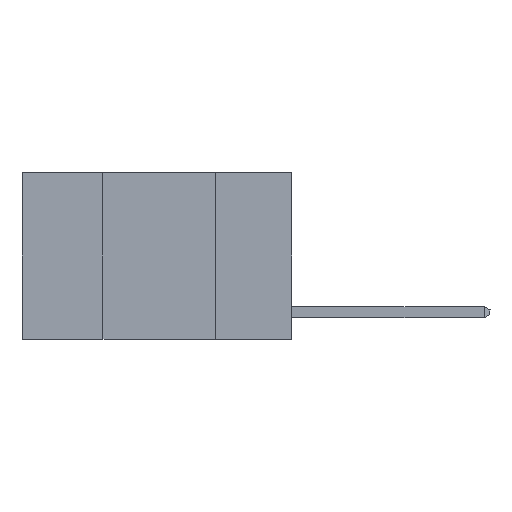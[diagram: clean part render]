
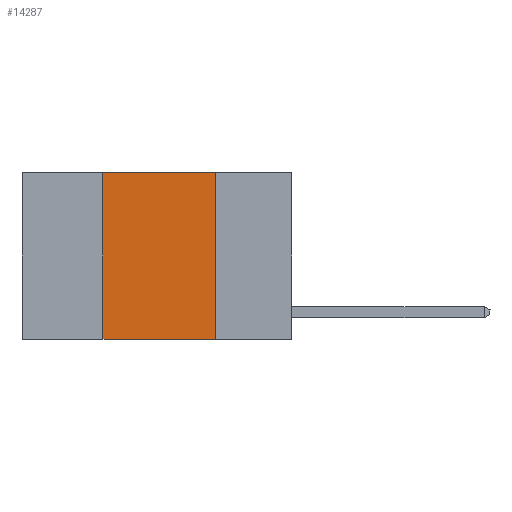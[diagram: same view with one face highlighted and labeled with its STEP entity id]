
A CAD part, left-side view. The second image highlights one B-rep face of the part: STEP entity #14287.
In plain terms, the highlighted planar face has unit normal (-1, 0, 0).
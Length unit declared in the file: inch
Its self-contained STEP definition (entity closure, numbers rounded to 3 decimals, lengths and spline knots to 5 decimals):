
#837 = EDGE_LOOP ( 'NONE', ( #17933, #16946, #6450, #17273 ) ) ;
#1262 = VECTOR ( 'NONE', #12781, 39.37008 ) ;
#1376 = VERTEX_POINT ( 'NONE', #6701 ) ;
#1674 = CARTESIAN_POINT ( 'NONE',  ( 0., 0.42, 0. ) ) ;
#2079 = DIRECTION ( 'NONE',  ( 0., -1., 0. ) ) ;
#2523 = DIRECTION ( 'NONE',  ( 0., -1., 0. ) ) ;
#2656 = VECTOR ( 'NONE', #2523, 39.37008 ) ;
#2995 = VERTEX_POINT ( 'NONE', #4851 ) ;
#3173 = CARTESIAN_POINT ( 'NONE',  ( 0., 0.6, 0. ) ) ;
#4442 = FACE_OUTER_BOUND ( 'NONE', #837, .T. ) ;
#4524 = CARTESIAN_POINT ( 'NONE',  ( 0., 0.17, 0. ) ) ;
#4851 = CARTESIAN_POINT ( 'NONE',  ( 0., 0.42, -0.37 ) ) ;
#4976 = EDGE_CURVE ( 'NONE', #19014, #17027, #4991, .T. ) ;
#4991 = LINE ( 'NONE', #10570, #2656 ) ;
#5814 = CARTESIAN_POINT ( 'NONE',  ( 0., 0.17, 0. ) ) ;
#6450 = ORIENTED_EDGE ( 'NONE', *, *, #12427, .F. ) ;
#6701 = CARTESIAN_POINT ( 'NONE',  ( 0., 0.17, -0.37 ) ) ;
#7117 = CARTESIAN_POINT ( 'NONE',  ( 0., 0.6, -0.37 ) ) ;
#7258 = DIRECTION ( 'NONE',  ( 0., 0., 1. ) ) ;
#8863 = AXIS2_PLACEMENT_3D ( 'NONE', #3173, #20954, #16207 ) ;
#8958 = EDGE_CURVE ( 'NONE', #2995, #1376, #20935, .T. ) ;
#10552 = CARTESIAN_POINT ( 'NONE',  ( 0., 0.42, 0. ) ) ;
#10570 = CARTESIAN_POINT ( 'NONE',  ( 0., 0.6, 0. ) ) ;
#12427 = EDGE_CURVE ( 'NONE', #2995, #19014, #14749, .T. ) ;
#12781 = DIRECTION ( 'NONE',  ( 0., 0., -1. ) ) ;
#13380 = VECTOR ( 'NONE', #7258, 39.37008 ) ;
#14287 = ADVANCED_FACE ( 'NONE', ( #4442 ), #14468, .F. ) ;
#14468 = PLANE ( 'NONE',  #8863 ) ;
#14749 = LINE ( 'NONE', #10552, #13380 ) ;
#16207 = DIRECTION ( 'NONE',  ( 0., 0., -1. ) ) ;
#16946 = ORIENTED_EDGE ( 'NONE', *, *, #4976, .F. ) ;
#17027 = VERTEX_POINT ( 'NONE', #5814 ) ;
#17273 = ORIENTED_EDGE ( 'NONE', *, *, #8958, .T. ) ;
#17933 = ORIENTED_EDGE ( 'NONE', *, *, #18273, .F. ) ;
#18273 = EDGE_CURVE ( 'NONE', #17027, #1376, #21293, .T. ) ;
#19014 = VERTEX_POINT ( 'NONE', #1674 ) ;
#20409 = VECTOR ( 'NONE', #2079, 39.37008 ) ;
#20935 = LINE ( 'NONE', #7117, #20409 ) ;
#20954 = DIRECTION ( 'NONE',  ( 1., 0., 0. ) ) ;
#21293 = LINE ( 'NONE', #4524, #1262 ) ;
